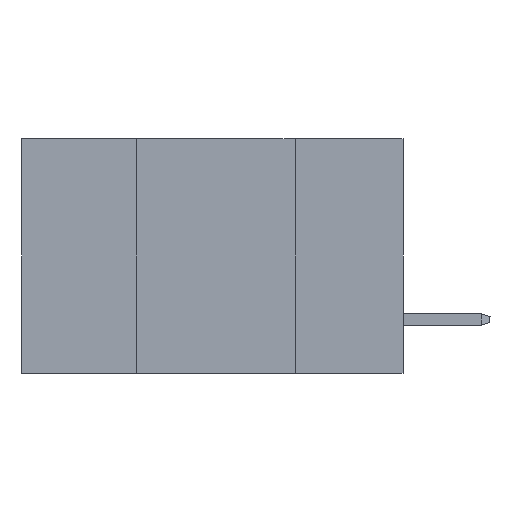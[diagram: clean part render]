
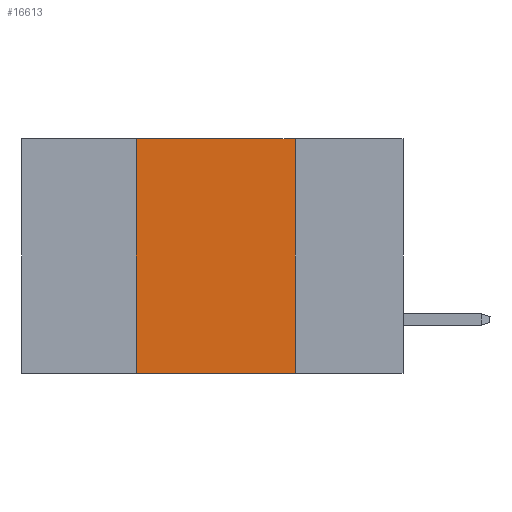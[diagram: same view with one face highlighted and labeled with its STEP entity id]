
A CAD part, left-side view. The second image highlights one B-rep face of the part: STEP entity #16613.
In plain terms, the highlighted planar face has unit normal (-1, 0, 0).
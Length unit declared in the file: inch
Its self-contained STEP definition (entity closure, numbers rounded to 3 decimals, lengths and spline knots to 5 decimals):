
#29 = DIRECTION ( 'NONE',  ( 0., 0., -1. ) ) ;
#68 = CARTESIAN_POINT ( 'NONE',  ( 0., 0.6, 0. ) ) ;
#701 = CARTESIAN_POINT ( 'NONE',  ( 0., 0.42, 0. ) ) ;
#721 = CARTESIAN_POINT ( 'NONE',  ( 0., 0.17, -0.37 ) ) ;
#1041 = LINE ( 'NONE', #701, #20419 ) ;
#1355 = EDGE_LOOP ( 'NONE', ( #18739, #18726, #18850, #19577 ) ) ;
#1639 = LINE ( 'NONE', #6872, #18431 ) ;
#1679 = VERTEX_POINT ( 'NONE', #18252 ) ;
#4665 = DIRECTION ( 'NONE',  ( 0., 0., -1. ) ) ;
#5044 = LINE ( 'NONE', #68, #14038 ) ;
#5459 = CARTESIAN_POINT ( 'NONE',  ( 0., 0.6, -0.37 ) ) ;
#5472 = VERTEX_POINT ( 'NONE', #5529 ) ;
#5529 = CARTESIAN_POINT ( 'NONE',  ( 0., 0.42, 0. ) ) ;
#6217 = EDGE_CURVE ( 'NONE', #21737, #7992, #1639, .T. ) ;
#6872 = CARTESIAN_POINT ( 'NONE',  ( 0., 0.17, 0. ) ) ;
#7796 = DIRECTION ( 'NONE',  ( 0., 0., 1. ) ) ;
#7963 = DIRECTION ( 'NONE',  ( 1., 0., 0. ) ) ;
#7992 = VERTEX_POINT ( 'NONE', #721 ) ;
#9697 = PLANE ( 'NONE',  #20517 ) ;
#10059 = CARTESIAN_POINT ( 'NONE',  ( 0., 0.6, 0. ) ) ;
#10128 = EDGE_CURVE ( 'NONE', #5472, #21737, #5044, .T. ) ;
#12233 = VECTOR ( 'NONE', #12638, 39.37008 ) ;
#12638 = DIRECTION ( 'NONE',  ( 0., -1., 0. ) ) ;
#14038 = VECTOR ( 'NONE', #16642, 39.37008 ) ;
#15251 = FACE_OUTER_BOUND ( 'NONE', #1355, .T. ) ;
#16613 = ADVANCED_FACE ( 'NONE', ( #15251 ), #9697, .F. ) ;
#16642 = DIRECTION ( 'NONE',  ( 0., -1., 0. ) ) ;
#17471 = EDGE_CURVE ( 'NONE', #1679, #5472, #1041, .T. ) ;
#18252 = CARTESIAN_POINT ( 'NONE',  ( 0., 0.42, -0.37 ) ) ;
#18431 = VECTOR ( 'NONE', #29, 39.37008 ) ;
#18619 = EDGE_CURVE ( 'NONE', #1679, #7992, #21556, .T. ) ;
#18726 = ORIENTED_EDGE ( 'NONE', *, *, #10128, .F. ) ;
#18739 = ORIENTED_EDGE ( 'NONE', *, *, #6217, .F. ) ;
#18850 = ORIENTED_EDGE ( 'NONE', *, *, #17471, .F. ) ;
#19124 = CARTESIAN_POINT ( 'NONE',  ( 0., 0.17, 0. ) ) ;
#19577 = ORIENTED_EDGE ( 'NONE', *, *, #18619, .T. ) ;
#20419 = VECTOR ( 'NONE', #7796, 39.37008 ) ;
#20517 = AXIS2_PLACEMENT_3D ( 'NONE', #10059, #7963, #4665 ) ;
#21556 = LINE ( 'NONE', #5459, #12233 ) ;
#21737 = VERTEX_POINT ( 'NONE', #19124 ) ;
